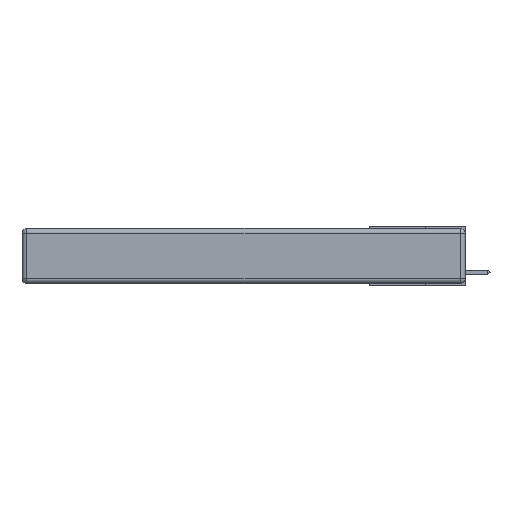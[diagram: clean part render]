
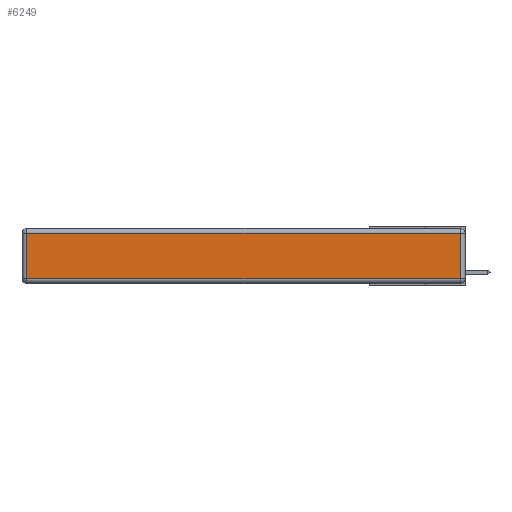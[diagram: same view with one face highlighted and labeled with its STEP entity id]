
A CAD part, left-side view. The second image highlights one B-rep face of the part: STEP entity #6249.
In plain terms, the highlighted planar face has unit normal (-1, 0, 0).
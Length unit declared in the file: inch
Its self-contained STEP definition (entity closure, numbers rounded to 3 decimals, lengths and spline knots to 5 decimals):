
#27 = CARTESIAN_POINT ( 'NONE',  ( 0., 2.72, -0.03 ) ) ;
#67 = LINE ( 'NONE', #7445, #2463 ) ;
#784 = EDGE_CURVE ( 'NONE', #2624, #9849, #1363, .T. ) ;
#1363 = LINE ( 'NONE', #7745, #2577 ) ;
#1532 = CARTESIAN_POINT ( 'NONE',  ( 0., 2.72, -0.343 ) ) ;
#1928 = VERTEX_POINT ( 'NONE', #27 ) ;
#2076 = DIRECTION ( 'NONE',  ( 0., 0., 1. ) ) ;
#2105 = VERTEX_POINT ( 'NONE', #10146 ) ;
#2463 = VECTOR ( 'NONE', #9379, 39.37008 ) ;
#2577 = VECTOR ( 'NONE', #2076, 39.37008 ) ;
#2624 = VERTEX_POINT ( 'NONE', #12428 ) ;
#3450 = ORIENTED_EDGE ( 'NONE', *, *, #8439, .T. ) ;
#3846 = PLANE ( 'NONE',  #6501 ) ;
#3959 = CARTESIAN_POINT ( 'NONE',  ( 0., 0., -0.343 ) ) ;
#4009 = FACE_OUTER_BOUND ( 'NONE', #12078, .T. ) ;
#4388 = DIRECTION ( 'NONE',  ( 0., 0., -1. ) ) ;
#4494 = ORIENTED_EDGE ( 'NONE', *, *, #5116, .T. ) ;
#5116 = EDGE_CURVE ( 'NONE', #2105, #2624, #67, .T. ) ;
#5511 = VECTOR ( 'NONE', #4388, 39.37008 ) ;
#5615 = LINE ( 'NONE', #10071, #8055 ) ;
#6146 = EDGE_CURVE ( 'NONE', #1928, #2105, #6583, .T. ) ;
#6249 = ADVANCED_FACE ( 'NONE', ( #4009 ), #3846, .T. ) ;
#6353 = ORIENTED_EDGE ( 'NONE', *, *, #784, .T. ) ;
#6501 = AXIS2_PLACEMENT_3D ( 'NONE', #3959, #9717, #8798 ) ;
#6583 = LINE ( 'NONE', #1532, #5511 ) ;
#7445 = CARTESIAN_POINT ( 'NONE',  ( 0., 0., -0.313 ) ) ;
#7745 = CARTESIAN_POINT ( 'NONE',  ( 0., 0.03, -0.343 ) ) ;
#8055 = VECTOR ( 'NONE', #12025, 39.37008 ) ;
#8439 = EDGE_CURVE ( 'NONE', #9849, #1928, #5615, .T. ) ;
#8798 = DIRECTION ( 'NONE',  ( 0., 0., 1. ) ) ;
#9379 = DIRECTION ( 'NONE',  ( 0., -1., 0. ) ) ;
#9456 = CARTESIAN_POINT ( 'NONE',  ( 0., 0.03, -0.03 ) ) ;
#9717 = DIRECTION ( 'NONE',  ( -1., 0., 0. ) ) ;
#9849 = VERTEX_POINT ( 'NONE', #9456 ) ;
#10071 = CARTESIAN_POINT ( 'NONE',  ( 0., 2.75, -0.03 ) ) ;
#10146 = CARTESIAN_POINT ( 'NONE',  ( 0., 2.72, -0.313 ) ) ;
#11237 = ORIENTED_EDGE ( 'NONE', *, *, #6146, .T. ) ;
#12025 = DIRECTION ( 'NONE',  ( 0., 1., 0. ) ) ;
#12078 = EDGE_LOOP ( 'NONE', ( #4494, #6353, #3450, #11237 ) ) ;
#12428 = CARTESIAN_POINT ( 'NONE',  ( 0., 0.03, -0.313 ) ) ;
